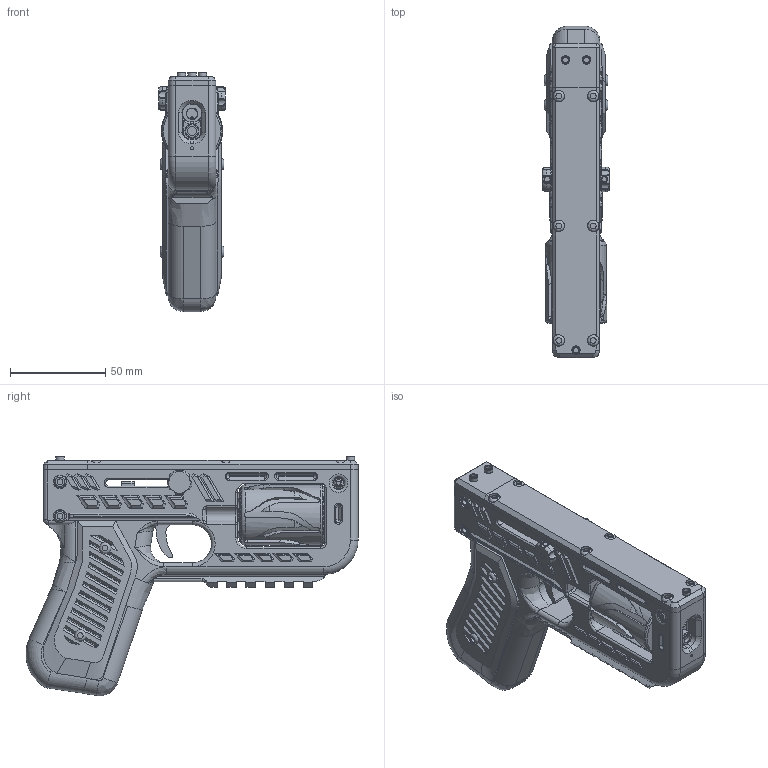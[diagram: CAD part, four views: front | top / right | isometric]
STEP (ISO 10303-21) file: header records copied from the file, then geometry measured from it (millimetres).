
FILE_DESCRIPTION(/* description */ (''),/* implementation_level */ '2;1');
FILE_NAME(/* name */ 'MaverickV2.4.stp',/* time_stamp */ '2020-11-10T10:23:28-06:00',/* author */ (''),/* organization */ (''),/* preprocessor_version */ 'ST-DEVELOPER v15.2',/* originating_system */ 'Autodesk Translator Framework v2.0.0.5431',/* authorisation */ '');
FILE_SCHEMA (('AUTOMOTIVE_DESIGN { 1 0 10303 214 3 1 1 }'));
Products named in the file (1): MaverickV2.4
Bounding box: 34.99 x 173.87 x 125.5 mm (x, y, z)
Volume: 255030.6 mm3; surface area: 19667403.7 mm2
Topology: 37 solids, 37 shells, 1908 faces, 4846 edges, 3086 vertices
Faces by surface type: plane 702, cylinder 484, bspline 436, torus 131, cone 124, sphere 31
Full cylindrical faces by diameter (mm): 1.8 x2, 2.75 x2, 2.8 x11, 2.9 x14, 3 x35, 3.1 x6, 3.2 x6, 3.5 x2, 4.4 x4, 4.497 x1, 4.831 x1, 5.1 x1, 6 x18, 7 x2, 7.3 x4, 7.33 x1, 32 x1
Entity records: 76660 total; most frequent: CARTESIAN_POINT 34459, ORIENTED_EDGE 9288, DIRECTION 7551, EDGE_CURVE 4644, VERTEX_POINT 3061, AXIS2_PLACEMENT_3D 2926, EDGE_LOOP 2253, ADVANCED_FACE 1908
